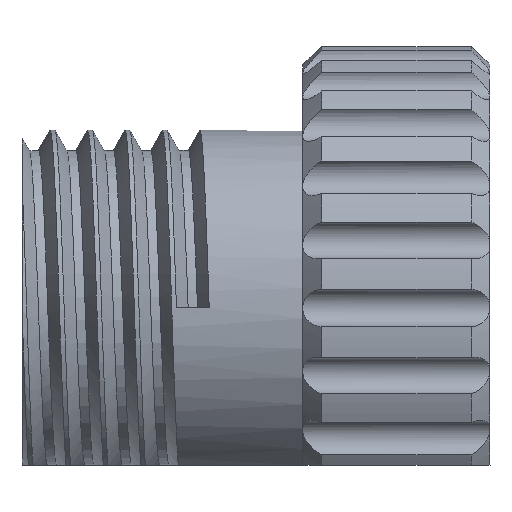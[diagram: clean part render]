
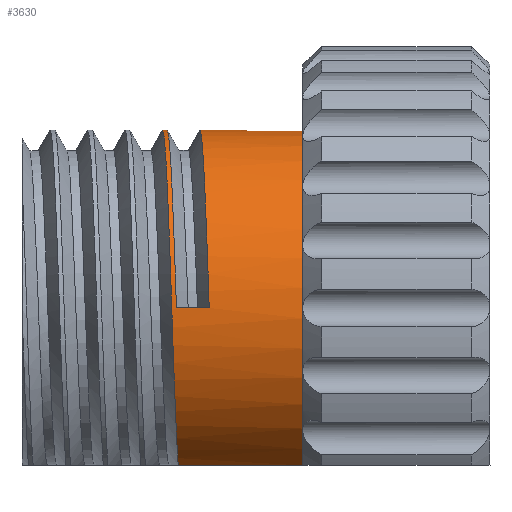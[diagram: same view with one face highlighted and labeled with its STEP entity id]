
A CAD part, left-side view. The second image highlights one B-rep face of the part: STEP entity #3630.
In plain terms, the highlighted cylindrical face has radius 6.032 mm (diameter 12.065 mm), a partial arc.
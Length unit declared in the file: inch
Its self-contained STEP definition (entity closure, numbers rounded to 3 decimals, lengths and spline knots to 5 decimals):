
#55 =( BOUNDED_CURVE ( )  B_SPLINE_CURVE ( 2, ( #1581, #3639, #6341, #6860, #2122, #4209, #5212, #2037, #1025, #6794, #3658, #5416, #6362, #4344, #6452, #97, #1651 ),
 .UNSPECIFIED., .F., .T. ) 
 B_SPLINE_CURVE_WITH_KNOTS ( ( 3, 2, 2, 2, 2, 2, 2, 2, 3 ),
 ( 0.57527, 0.58333, 0.60417, 0.625, 0.64583, 0.66667, 0.6875, 0.70833, 0.7164 ),
 .UNSPECIFIED. ) 
 CURVE ( )  GEOMETRIC_REPRESENTATION_ITEM ( )  RATIONAL_B_SPLINE_CURVE ( ( 0.964, 0.971, 1., 0.924, 1., 0.924, 1., 0.924, 1., 0.924, 1., 0.924, 1., 0.924, 1., 0.971, 0.964 ) ) 
 REPRESENTATION_ITEM ( '' )  );
#97 = CARTESIAN_POINT ( 'NONE',  ( -0.1423, 0.1676, -0.19358 ) ) ;
#105 = ORIENTED_EDGE ( 'NONE', *, *, #1778, .T. ) ;
#149 = DIRECTION ( 'NONE',  ( 0., 1., 0. ) ) ;
#173 = LINE ( 'NONE', #5991, #2006 ) ;
#309 = DIRECTION ( 'NONE',  ( 0., 0., 1. ) ) ;
#425 = CARTESIAN_POINT ( 'NONE',  ( 0.16794, 0.15625, -0.16794 ) ) ;
#553 = DIRECTION ( 'NONE',  ( 0., -1., 0. ) ) ;
#771 = LINE ( 'NONE', #3558, #4503 ) ;
#861 = CARTESIAN_POINT ( 'NONE',  ( -0.2375, 0.12813, 0.09838 ) ) ;
#879 = CARTESIAN_POINT ( 'NONE',  ( 0.11017, 0.375, -0.2104 ) ) ;
#951 = CARTESIAN_POINT ( 'NONE',  ( -0.16794, 0.175, 0.16794 ) ) ;
#974 = CARTESIAN_POINT ( 'NONE',  ( -0.2375, 0.125, 0. ) ) ;
#976 = EDGE_CURVE ( 'NONE', #5831, #6391, #173, .T. ) ;
#993 = CARTESIAN_POINT ( 'NONE',  ( 0.2375, 0.19063, 0.09838 ) ) ;
#1025 = CARTESIAN_POINT ( 'NONE',  ( 0., 0.1875, 0.2375 ) ) ;
#1040 = CARTESIAN_POINT ( 'NONE',  ( 0.11017, 0.20239, -0.2104 ) ) ;
#1492 = CYLINDRICAL_SURFACE ( 'NONE', #2840, 0.2375 ) ;
#1568 = FACE_OUTER_BOUND ( 'NONE', #6216, .T. ) ;
#1581 = CARTESIAN_POINT ( 'NONE',  ( 0.11017, 0.20864, -0.2104 ) ) ;
#1634 = DIRECTION ( 'NONE',  ( 0., 0., -1. ) ) ;
#1651 = CARTESIAN_POINT ( 'NONE',  ( -0.11017, 0.16636, -0.2104 ) ) ;
#1653 =( BOUNDED_CURVE ( )  B_SPLINE_CURVE ( 2, ( #6122, #4546, #425, #5069, #3694, #5250, #2431, #2967, #2601, #5210, #6652, #861, #974 ),
 .UNSPECIFIED., .F., .F. ) 
 B_SPLINE_CURVE_WITH_KNOTS ( ( 3, 2, 2, 2, 2, 2, 3 ),
 ( 0.74193, 0.75, 0.77083, 0.79167, 0.8125, 0.83333, 0.85417 ),
 .UNSPECIFIED. ) 
 CURVE ( )  GEOMETRIC_REPRESENTATION_ITEM ( )  RATIONAL_B_SPLINE_CURVE ( ( 0.964, 0.971, 1., 0.924, 1., 0.924, 1., 0.924, 1., 0.924, 1., 0.924, 1. ) ) 
 REPRESENTATION_ITEM ( '' )  );
#1674 = VERTEX_POINT ( 'NONE', #5118 ) ;
#1716 = CARTESIAN_POINT ( 'NONE',  ( 0.11017, 0.15864, -0.2104 ) ) ;
#1778 = EDGE_CURVE ( 'NONE', #1674, #4418, #55, .T. ) ;
#2006 = VECTOR ( 'NONE', #149, 39.37008 ) ;
#2037 = CARTESIAN_POINT ( 'NONE',  ( 0.09838, 0.19063, 0.2375 ) ) ;
#2104 = ORIENTED_EDGE ( 'NONE', *, *, #2892, .F. ) ;
#2122 = CARTESIAN_POINT ( 'NONE',  ( 0.2375, 0.2, 0. ) ) ;
#2137 = EDGE_CURVE ( 'NONE', #6780, #5831, #4751, .T. ) ;
#2177 = ORIENTED_EDGE ( 'NONE', *, *, #3624, .T. ) ;
#2181 = VERTEX_POINT ( 'NONE', #6059 ) ;
#2226 = DIRECTION ( 'NONE',  ( 0., -1., 0. ) ) ;
#2431 = CARTESIAN_POINT ( 'NONE',  ( 0.16794, 0.14375, 0.16794 ) ) ;
#2510 = VERTEX_POINT ( 'NONE', #4669 ) ;
#2579 = CARTESIAN_POINT ( 'NONE',  ( 0.1423, 0.20115, -0.19358 ) ) ;
#2601 = CARTESIAN_POINT ( 'NONE',  ( 0., 0.1375, 0.2375 ) ) ;
#2619 = CARTESIAN_POINT ( 'NONE',  ( 0.16794, 0.1875, 0.16794 ) ) ;
#2640 = CARTESIAN_POINT ( 'NONE',  ( -0.2375, 0.16875, 0. ) ) ;
#2716 = CARTESIAN_POINT ( 'NONE',  ( -0.11017, 0.375, -0.2104 ) ) ;
#2793 = EDGE_CURVE ( 'NONE', #5304, #2181, #771, .T. ) ;
#2840 = AXIS2_PLACEMENT_3D ( 'NONE', #5353, #2226, #1634 ) ;
#2892 = EDGE_CURVE ( 'NONE', #2510, #2181, #3485, .T. ) ;
#2967 = CARTESIAN_POINT ( 'NONE',  ( 0.09838, 0.14063, 0.2375 ) ) ;
#3356 = CARTESIAN_POINT ( 'NONE',  ( -0.2375, 0.125, 0. ) ) ;
#3485 =( BOUNDED_CURVE ( )  B_SPLINE_CURVE ( 2, ( #1040, #2579, #3669, #6282, #5206, #993, #2619, #4133, #5704, #5796, #951, #5182, #2640 ),
 .UNSPECIFIED., .F., .F. ) 
 B_SPLINE_CURVE_WITH_KNOTS ( ( 3, 2, 2, 2, 2, 2, 3 ),
 ( 0.74193, 0.75, 0.77083, 0.79167, 0.8125, 0.83333, 0.85417 ),
 .UNSPECIFIED. ) 
 CURVE ( )  GEOMETRIC_REPRESENTATION_ITEM ( )  RATIONAL_B_SPLINE_CURVE ( ( 0.964, 0.971, 1., 0.924, 1., 0.924, 1., 0.924, 1., 0.924, 1., 0.924, 1. ) ) 
 REPRESENTATION_ITEM ( '' )  );
#3558 = CARTESIAN_POINT ( 'NONE',  ( -0.2375, 0.375, 0. ) ) ;
#3624 = EDGE_CURVE ( 'NONE', #4418, #6780, #6449, .T. ) ;
#3630 = ADVANCED_FACE ( 'NONE', ( #1568 ), #1492, .T. ) ;
#3639 = CARTESIAN_POINT ( 'NONE',  ( 0.1423, 0.2074, -0.19358 ) ) ;
#3658 = CARTESIAN_POINT ( 'NONE',  ( -0.16794, 0.18125, 0.16794 ) ) ;
#3669 = CARTESIAN_POINT ( 'NONE',  ( 0.16794, 0.2, -0.16794 ) ) ;
#3670 = DIRECTION ( 'NONE',  ( 0., 1., 0. ) ) ;
#3694 = CARTESIAN_POINT ( 'NONE',  ( 0.2375, 0.15, 0. ) ) ;
#3870 = EDGE_CURVE ( 'NONE', #2510, #1674, #4715, .T. ) ;
#4133 = CARTESIAN_POINT ( 'NONE',  ( 0.09838, 0.18437, 0.2375 ) ) ;
#4209 = CARTESIAN_POINT ( 'NONE',  ( 0.2375, 0.19688, 0.09838 ) ) ;
#4275 = CARTESIAN_POINT ( 'NONE',  ( 0.11017, 0., -0.2104 ) ) ;
#4319 = AXIS2_PLACEMENT_3D ( 'NONE', #6437, #5087, #309 ) ;
#4344 = CARTESIAN_POINT ( 'NONE',  ( -0.2375, 0.17188, -0.09838 ) ) ;
#4418 = VERTEX_POINT ( 'NONE', #5174 ) ;
#4503 = VECTOR ( 'NONE', #5661, 39.37008 ) ;
#4546 = CARTESIAN_POINT ( 'NONE',  ( 0.1423, 0.1574, -0.19358 ) ) ;
#4562 = ORIENTED_EDGE ( 'NONE', *, *, #5677, .T. ) ;
#4669 = CARTESIAN_POINT ( 'NONE',  ( 0.11017, 0.20239, -0.2104 ) ) ;
#4715 = LINE ( 'NONE', #879, #5450 ) ;
#4751 = CIRCLE ( 'NONE', #4319, 0.2375 ) ;
#5010 = ORIENTED_EDGE ( 'NONE', *, *, #2137, .T. ) ;
#5069 = CARTESIAN_POINT ( 'NONE',  ( 0.2375, 0.15313, -0.09838 ) ) ;
#5087 = DIRECTION ( 'NONE',  ( 0., 1., 0. ) ) ;
#5118 = CARTESIAN_POINT ( 'NONE',  ( 0.11017, 0.20864, -0.2104 ) ) ;
#5174 = CARTESIAN_POINT ( 'NONE',  ( -0.11017, 0.16636, -0.2104 ) ) ;
#5182 = CARTESIAN_POINT ( 'NONE',  ( -0.2375, 0.17188, 0.09838 ) ) ;
#5206 = CARTESIAN_POINT ( 'NONE',  ( 0.2375, 0.19375, 0. ) ) ;
#5210 = CARTESIAN_POINT ( 'NONE',  ( -0.09838, 0.13438, 0.2375 ) ) ;
#5212 = CARTESIAN_POINT ( 'NONE',  ( 0.16794, 0.19375, 0.16794 ) ) ;
#5250 = CARTESIAN_POINT ( 'NONE',  ( 0.2375, 0.14688, 0.09838 ) ) ;
#5304 = VERTEX_POINT ( 'NONE', #3356 ) ;
#5353 = CARTESIAN_POINT ( 'NONE',  ( 0., 0.375, 0. ) ) ;
#5413 = ORIENTED_EDGE ( 'NONE', *, *, #3870, .T. ) ;
#5416 = CARTESIAN_POINT ( 'NONE',  ( -0.2375, 0.17813, 0.09838 ) ) ;
#5450 = VECTOR ( 'NONE', #3670, 39.37008 ) ;
#5661 = DIRECTION ( 'NONE',  ( 0., 1., 0. ) ) ;
#5677 = EDGE_CURVE ( 'NONE', #6391, #5304, #1653, .T. ) ;
#5704 = CARTESIAN_POINT ( 'NONE',  ( 0., 0.18125, 0.2375 ) ) ;
#5796 = CARTESIAN_POINT ( 'NONE',  ( -0.09838, 0.17812, 0.2375 ) ) ;
#5831 = VERTEX_POINT ( 'NONE', #4275 ) ;
#5991 = CARTESIAN_POINT ( 'NONE',  ( 0.11017, 0.375, -0.2104 ) ) ;
#6059 = CARTESIAN_POINT ( 'NONE',  ( -0.2375, 0.16875, 0. ) ) ;
#6122 = CARTESIAN_POINT ( 'NONE',  ( 0.11017, 0.15864, -0.2104 ) ) ;
#6216 = EDGE_LOOP ( 'NONE', ( #105, #2177, #5010, #6624, #4562, #6468, #2104, #5413 ) ) ;
#6282 = CARTESIAN_POINT ( 'NONE',  ( 0.2375, 0.19687, -0.09838 ) ) ;
#6341 = CARTESIAN_POINT ( 'NONE',  ( 0.16794, 0.20625, -0.16794 ) ) ;
#6362 = CARTESIAN_POINT ( 'NONE',  ( -0.2375, 0.175, 0. ) ) ;
#6391 = VERTEX_POINT ( 'NONE', #1716 ) ;
#6437 = CARTESIAN_POINT ( 'NONE',  ( 0., 0., 0. ) ) ;
#6449 = LINE ( 'NONE', #2716, #6677 ) ;
#6452 = CARTESIAN_POINT ( 'NONE',  ( -0.16794, 0.16875, -0.16794 ) ) ;
#6468 = ORIENTED_EDGE ( 'NONE', *, *, #2793, .T. ) ;
#6582 = CARTESIAN_POINT ( 'NONE',  ( -0.11017, 0., -0.2104 ) ) ;
#6624 = ORIENTED_EDGE ( 'NONE', *, *, #976, .T. ) ;
#6652 = CARTESIAN_POINT ( 'NONE',  ( -0.16794, 0.13125, 0.16794 ) ) ;
#6677 = VECTOR ( 'NONE', #553, 39.37008 ) ;
#6780 = VERTEX_POINT ( 'NONE', #6582 ) ;
#6794 = CARTESIAN_POINT ( 'NONE',  ( -0.09838, 0.18438, 0.2375 ) ) ;
#6860 = CARTESIAN_POINT ( 'NONE',  ( 0.2375, 0.20313, -0.09838 ) ) ;
